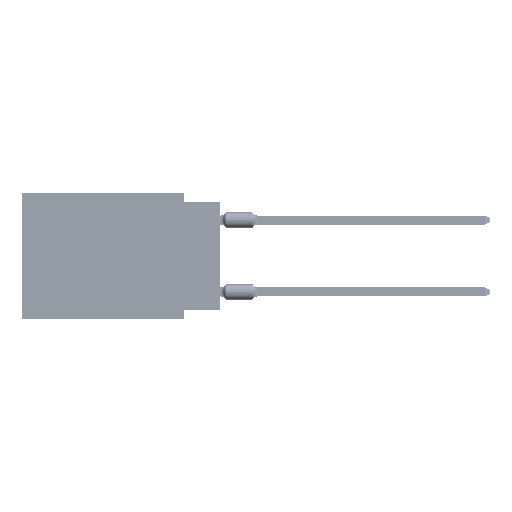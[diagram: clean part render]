
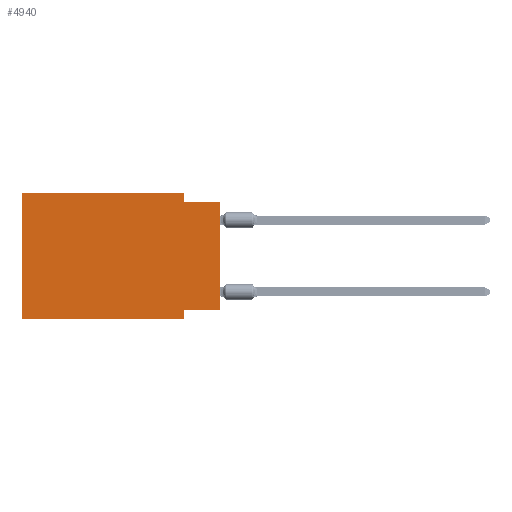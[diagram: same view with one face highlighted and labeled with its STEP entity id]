
A CAD part, left-side view. The second image highlights one B-rep face of the part: STEP entity #4940.
In plain terms, the highlighted planar face has unit normal (-1, 0, 0).
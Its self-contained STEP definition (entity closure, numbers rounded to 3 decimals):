
#2521 = DIRECTION ( 'NONE',  ( 0., -1., 0. ) ) ;
#4302 = EDGE_CURVE ( 'NONE', #80014, #86217, #76343, .T. ) ;
#4940 = ADVANCED_FACE ( 'NONE', ( #6320 ), #71363, .F. ) ;
#5049 = DIRECTION ( 'NONE',  ( 0., 0., 1. ) ) ;
#6179 = VECTOR ( 'NONE', #68417, 1000. ) ;
#6320 = FACE_OUTER_BOUND ( 'NONE', #46829, .T. ) ;
#8425 = VERTEX_POINT ( 'NONE', #50352 ) ;
#9584 = EDGE_CURVE ( 'NONE', #24885, #78456, #35841, .T. ) ;
#10679 = VECTOR ( 'NONE', #49493, 1000. ) ;
#10808 = EDGE_CURVE ( 'NONE', #86191, #8425, #22120, .T. ) ;
#14908 = LINE ( 'NONE', #80467, #57425 ) ;
#16167 = LINE ( 'NONE', #47911, #10679 ) ;
#17352 = CARTESIAN_POINT ( 'NONE',  ( 0., 13.97, 0. ) ) ;
#19602 = ORIENTED_EDGE ( 'NONE', *, *, #40432, .F. ) ;
#22120 = LINE ( 'NONE', #97307, #66232 ) ;
#24005 = DIRECTION ( 'NONE',  ( 1., 0., 0. ) ) ;
#24172 = ORIENTED_EDGE ( 'NONE', *, *, #10808, .F. ) ;
#24869 = VECTOR ( 'NONE', #52662, 1000. ) ;
#24885 = VERTEX_POINT ( 'NONE', #32520 ) ;
#27027 = CARTESIAN_POINT ( 'NONE',  ( 0., 2.54, 0. ) ) ;
#29232 = ORIENTED_EDGE ( 'NONE', *, *, #66890, .T. ) ;
#31550 = CARTESIAN_POINT ( 'NONE',  ( 0., 13.97, 0. ) ) ;
#31744 = DIRECTION ( 'NONE',  ( 0., -1., 0. ) ) ;
#31901 = AXIS2_PLACEMENT_3D ( 'NONE', #31550, #24005, #64348 ) ;
#32520 = CARTESIAN_POINT ( 'NONE',  ( 0., 2.54, -0.635 ) ) ;
#33897 = CARTESIAN_POINT ( 'NONE',  ( 0., 13.97, -8.89 ) ) ;
#34367 = ORIENTED_EDGE ( 'NONE', *, *, #69820, .F. ) ;
#35151 = EDGE_CURVE ( 'NONE', #80014, #86191, #85130, .T. ) ;
#35612 = CARTESIAN_POINT ( 'NONE',  ( 0., 2.54, -8.89 ) ) ;
#35841 = LINE ( 'NONE', #58974, #60964 ) ;
#40432 = EDGE_CURVE ( 'NONE', #93050, #86217, #16167, .T. ) ;
#46564 = ORIENTED_EDGE ( 'NONE', *, *, #35151, .F. ) ;
#46829 = EDGE_LOOP ( 'NONE', ( #29232, #71471, #34367, #24172, #46564, #93224, #19602, #55237 ) ) ;
#47283 = CARTESIAN_POINT ( 'NONE',  ( 0., 0., -8.255 ) ) ;
#47911 = CARTESIAN_POINT ( 'NONE',  ( 0., 2.54, -8.89 ) ) ;
#49493 = DIRECTION ( 'NONE',  ( 0., 0., -1. ) ) ;
#50352 = CARTESIAN_POINT ( 'NONE',  ( 0., 2.54, 0. ) ) ;
#50742 = CARTESIAN_POINT ( 'NONE',  ( 0., 13.97, -8.89 ) ) ;
#52662 = DIRECTION ( 'NONE',  ( 0., 1., 0. ) ) ;
#55237 = ORIENTED_EDGE ( 'NONE', *, *, #68684, .F. ) ;
#57425 = VECTOR ( 'NONE', #90631, 1000. ) ;
#58974 = CARTESIAN_POINT ( 'NONE',  ( 0., 0., -0.635 ) ) ;
#60202 = CARTESIAN_POINT ( 'NONE',  ( 0., 0., -8.255 ) ) ;
#60964 = VECTOR ( 'NONE', #2521, 1000. ) ;
#64348 = DIRECTION ( 'NONE',  ( 0., 0., -1. ) ) ;
#66232 = VECTOR ( 'NONE', #31744, 1000. ) ;
#66575 = VECTOR ( 'NONE', #5049, 1000. ) ;
#66890 = EDGE_CURVE ( 'NONE', #86899, #78456, #14908, .T. ) ;
#68417 = DIRECTION ( 'NONE',  ( 0., 0., -1. ) ) ;
#68684 = EDGE_CURVE ( 'NONE', #86899, #93050, #93506, .T. ) ;
#69820 = EDGE_CURVE ( 'NONE', #8425, #24885, #75423, .T. ) ;
#71363 = PLANE ( 'NONE',  #31901 ) ;
#71471 = ORIENTED_EDGE ( 'NONE', *, *, #9584, .F. ) ;
#75423 = LINE ( 'NONE', #27027, #6179 ) ;
#75481 = CARTESIAN_POINT ( 'NONE',  ( 0., 0., -0.635 ) ) ;
#76343 = LINE ( 'NONE', #33897, #100725 ) ;
#78456 = VERTEX_POINT ( 'NONE', #75481 ) ;
#80014 = VERTEX_POINT ( 'NONE', #50742 ) ;
#80467 = CARTESIAN_POINT ( 'NONE',  ( 0., 0., 0. ) ) ;
#81241 = CARTESIAN_POINT ( 'NONE',  ( 0., 2.54, -8.255 ) ) ;
#85130 = LINE ( 'NONE', #95337, #66575 ) ;
#86191 = VERTEX_POINT ( 'NONE', #17352 ) ;
#86217 = VERTEX_POINT ( 'NONE', #35612 ) ;
#86899 = VERTEX_POINT ( 'NONE', #47283 ) ;
#90631 = DIRECTION ( 'NONE',  ( 0., 0., 1. ) ) ;
#93050 = VERTEX_POINT ( 'NONE', #81241 ) ;
#93224 = ORIENTED_EDGE ( 'NONE', *, *, #4302, .T. ) ;
#93506 = LINE ( 'NONE', #60202, #24869 ) ;
#95337 = CARTESIAN_POINT ( 'NONE',  ( 0., 13.97, 0. ) ) ;
#97307 = CARTESIAN_POINT ( 'NONE',  ( 0., 13.97, 0. ) ) ;
#100517 = DIRECTION ( 'NONE',  ( 0., -1., 0. ) ) ;
#100725 = VECTOR ( 'NONE', #100517, 1000. ) ;
